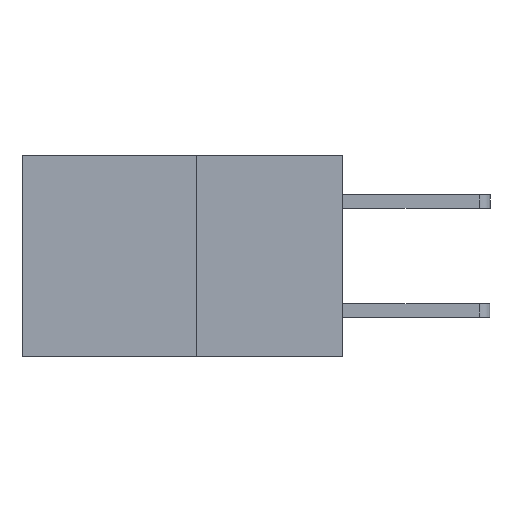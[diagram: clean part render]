
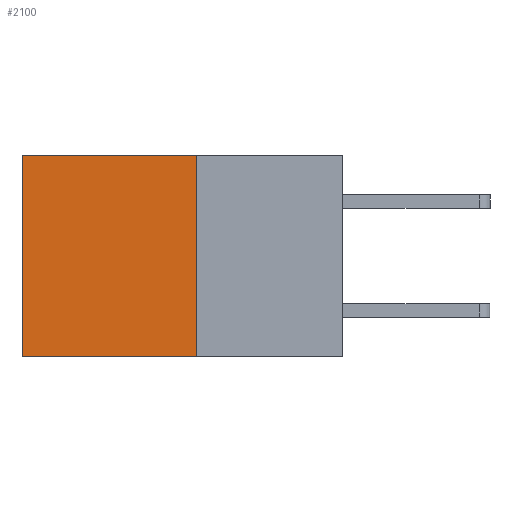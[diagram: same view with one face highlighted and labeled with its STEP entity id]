
A CAD part, left-side view. The second image highlights one B-rep face of the part: STEP entity #2100.
In plain terms, the highlighted planar face has unit normal (-1, 0, 0).
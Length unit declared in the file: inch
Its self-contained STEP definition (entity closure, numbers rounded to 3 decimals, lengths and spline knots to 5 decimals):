
#166 = CARTESIAN_POINT ( 'NONE',  ( 0.277, 0.59, -0.37 ) ) ;
#216 = DIRECTION ( 'NONE',  ( 0., 0., -1. ) ) ;
#474 = CARTESIAN_POINT ( 'NONE',  ( 0.277, 0.27, 0. ) ) ;
#625 = ORIENTED_EDGE ( 'NONE', *, *, #6258, .T. ) ;
#720 = CARTESIAN_POINT ( 'NONE',  ( 0.277, 0.27, -0.37 ) ) ;
#817 = ORIENTED_EDGE ( 'NONE', *, *, #2094, .F. ) ;
#1270 = LINE ( 'NONE', #166, #8657 ) ;
#1536 = CARTESIAN_POINT ( 'NONE',  ( 0.277, 0.59, 0. ) ) ;
#1602 = CARTESIAN_POINT ( 'NONE',  ( 0.277, 0.27, -0.37 ) ) ;
#1875 = DIRECTION ( 'NONE',  ( 0., 0., -1. ) ) ;
#2094 = EDGE_CURVE ( 'NONE', #7176, #3471, #6103, .T. ) ;
#2100 = ADVANCED_FACE ( 'NONE', ( #7928 ), #2471, .F. ) ;
#2471 = PLANE ( 'NONE',  #7007 ) ;
#3163 = ORIENTED_EDGE ( 'NONE', *, *, #8858, .F. ) ;
#3471 = VERTEX_POINT ( 'NONE', #4874 ) ;
#3515 = LINE ( 'NONE', #474, #7010 ) ;
#4160 = CARTESIAN_POINT ( 'NONE',  ( 0.277, 0.27, -0.37 ) ) ;
#4186 = CARTESIAN_POINT ( 'NONE',  ( 0.277, 0.27, 0. ) ) ;
#4260 = VECTOR ( 'NONE', #7290, 39.37008 ) ;
#4418 = VERTEX_POINT ( 'NONE', #1536 ) ;
#4874 = CARTESIAN_POINT ( 'NONE',  ( 0.277, 0.59, -0.37 ) ) ;
#5175 = DIRECTION ( 'NONE',  ( 0., 0., -1. ) ) ;
#5276 = VECTOR ( 'NONE', #216, 39.37008 ) ;
#5519 = VERTEX_POINT ( 'NONE', #4186 ) ;
#5652 = EDGE_LOOP ( 'NONE', ( #625, #817, #3163, #8692 ) ) ;
#5686 = DIRECTION ( 'NONE',  ( 1., 0., 0. ) ) ;
#6038 = EDGE_CURVE ( 'NONE', #5519, #4418, #3515, .T. ) ;
#6103 = LINE ( 'NONE', #4160, #4260 ) ;
#6258 = EDGE_CURVE ( 'NONE', #4418, #3471, #1270, .T. ) ;
#7007 = AXIS2_PLACEMENT_3D ( 'NONE', #720, #5686, #1875 ) ;
#7010 = VECTOR ( 'NONE', #8168, 39.37008 ) ;
#7098 = LINE ( 'NONE', #1602, #5276 ) ;
#7176 = VERTEX_POINT ( 'NONE', #8148 ) ;
#7290 = DIRECTION ( 'NONE',  ( 0., 1., 0. ) ) ;
#7928 = FACE_OUTER_BOUND ( 'NONE', #5652, .T. ) ;
#8148 = CARTESIAN_POINT ( 'NONE',  ( 0.277, 0.27, -0.37 ) ) ;
#8168 = DIRECTION ( 'NONE',  ( 0., 1., 0. ) ) ;
#8657 = VECTOR ( 'NONE', #5175, 39.37008 ) ;
#8692 = ORIENTED_EDGE ( 'NONE', *, *, #6038, .T. ) ;
#8858 = EDGE_CURVE ( 'NONE', #5519, #7176, #7098, .T. ) ;
